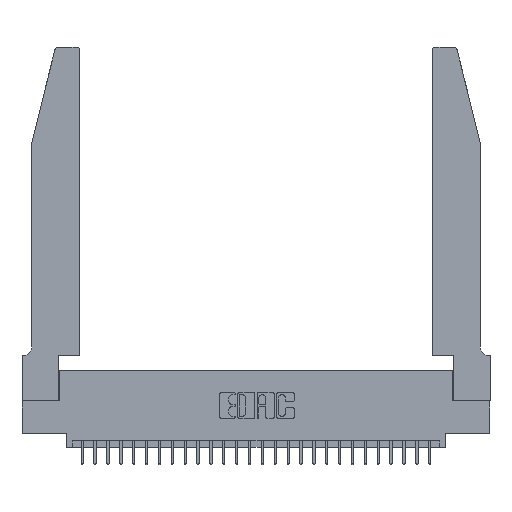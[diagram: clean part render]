
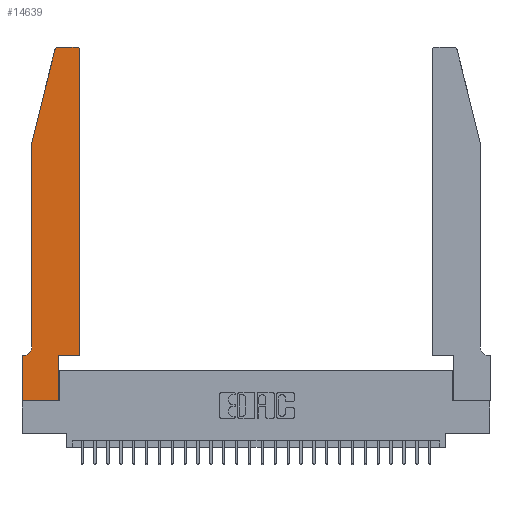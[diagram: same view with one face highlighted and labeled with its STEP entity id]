
A CAD part, top view. The second image highlights one B-rep face of the part: STEP entity #14639.
In plain terms, the highlighted planar face has unit normal (0, 0, 1).
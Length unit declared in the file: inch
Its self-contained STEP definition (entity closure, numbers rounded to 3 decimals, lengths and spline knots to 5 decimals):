
#9 = EDGE_CURVE ( 'NONE', #318, #7295, #23591, .T. ) ;
#57 = CARTESIAN_POINT ( 'NONE',  ( 0., 0.35, 0.37 ) ) ;
#318 = VERTEX_POINT ( 'NONE', #835 ) ;
#504 = DIRECTION ( 'NONE',  ( 1., 0., 0. ) ) ;
#835 = CARTESIAN_POINT ( 'NONE',  ( 0., 0.35, 0.37 ) ) ;
#884 = VERTEX_POINT ( 'NONE', #5884 ) ;
#1774 = LINE ( 'NONE', #19992, #11180 ) ;
#2488 = EDGE_CURVE ( 'NONE', #14502, #18545, #19866, .T. ) ;
#2671 = AXIS2_PLACEMENT_3D ( 'NONE', #21023, #7604, #20881 ) ;
#3238 = DIRECTION ( 'NONE',  ( 0., 1., 0. ) ) ;
#4235 = ORIENTED_EDGE ( 'NONE', *, *, #9, .T. ) ;
#4364 = DIRECTION ( 'NONE',  ( 1., 0., 0. ) ) ;
#4468 = ORIENTED_EDGE ( 'NONE', *, *, #12626, .T. ) ;
#4615 = EDGE_LOOP ( 'NONE', ( #11640, #15541, #27743, #25174, #7174, #15410, #4235, #6687, #4654, #4468, #18654, #24022 ) ) ;
#4654 = ORIENTED_EDGE ( 'NONE', *, *, #25054, .T. ) ;
#5324 = CARTESIAN_POINT ( 'NONE',  ( 0.4505, 0.35, 0.37 ) ) ;
#5884 = CARTESIAN_POINT ( 'NONE',  ( 0.0755, 2., 0.37 ) ) ;
#6075 = EDGE_CURVE ( 'NONE', #17084, #14502, #9820, .T. ) ;
#6185 = CARTESIAN_POINT ( 'NONE',  ( 0.4505, 2.72, 0.37 ) ) ;
#6214 = CARTESIAN_POINT ( 'NONE',  ( 0.0755, 2., 0.37 ) ) ;
#6383 = VERTEX_POINT ( 'NONE', #20259 ) ;
#6635 = CARTESIAN_POINT ( 'NONE',  ( 0.0055, 0.42, 0.37 ) ) ;
#6687 = ORIENTED_EDGE ( 'NONE', *, *, #10518, .T. ) ;
#6731 = VECTOR ( 'NONE', #17274, 39.37008 ) ;
#6787 = AXIS2_PLACEMENT_3D ( 'NONE', #57, #11114, #504 ) ;
#7174 = ORIENTED_EDGE ( 'NONE', *, *, #16550, .T. ) ;
#7295 = VERTEX_POINT ( 'NONE', #9009 ) ;
#7604 = DIRECTION ( 'NONE',  ( 0., 0., 1. ) ) ;
#8099 = CARTESIAN_POINT ( 'NONE',  ( 0.2865, 0.35, 0.37 ) ) ;
#8290 = LINE ( 'NONE', #14444, #14139 ) ;
#9009 = CARTESIAN_POINT ( 'NONE',  ( 0., 0., 0.37 ) ) ;
#9427 = VECTOR ( 'NONE', #4364, 39.37008 ) ;
#9759 = VERTEX_POINT ( 'NONE', #22353 ) ;
#9820 = LINE ( 'NONE', #20915, #17153 ) ;
#10478 = DIRECTION ( 'NONE',  ( -1., 0., 0. ) ) ;
#10518 = EDGE_CURVE ( 'NONE', #7295, #13391, #16001, .T. ) ;
#10576 = LINE ( 'NONE', #6214, #6731 ) ;
#10853 = DIRECTION ( 'NONE',  ( -1., 0., 0. ) ) ;
#11114 = DIRECTION ( 'NONE',  ( 0., 0., 1. ) ) ;
#11180 = VECTOR ( 'NONE', #22343, 39.37008 ) ;
#11543 = FACE_OUTER_BOUND ( 'NONE', #4615, .T. ) ;
#11640 = ORIENTED_EDGE ( 'NONE', *, *, #18376, .T. ) ;
#11825 = DIRECTION ( 'NONE',  ( 0., -1., 0. ) ) ;
#12626 = EDGE_CURVE ( 'NONE', #15548, #17084, #13453, .T. ) ;
#12737 = DIRECTION ( 'NONE',  ( 0., 0., -1. ) ) ;
#13391 = VERTEX_POINT ( 'NONE', #22506 ) ;
#13453 = LINE ( 'NONE', #26604, #26737 ) ;
#13742 = LINE ( 'NONE', #27337, #27738 ) ;
#13824 = CARTESIAN_POINT ( 'NONE',  ( 0., 0., 0.37 ) ) ;
#14139 = VECTOR ( 'NONE', #10478, 39.37008 ) ;
#14385 = DIRECTION ( 'NONE',  ( 1., 0., 0. ) ) ;
#14428 = CARTESIAN_POINT ( 'NONE',  ( 0.2865, 0.35, 0.37 ) ) ;
#14435 = CIRCLE ( 'NONE', #19531, 0.03 ) ;
#14444 = CARTESIAN_POINT ( 'NONE',  ( 0.0755, 0.35, 0.37 ) ) ;
#14502 = VERTEX_POINT ( 'NONE', #6185 ) ;
#14639 = ADVANCED_FACE ( 'NONE', ( #11543 ), #20466, .T. ) ;
#15410 = ORIENTED_EDGE ( 'NONE', *, *, #21966, .T. ) ;
#15460 = EDGE_CURVE ( 'NONE', #9759, #19875, #14435, .T. ) ;
#15541 = ORIENTED_EDGE ( 'NONE', *, *, #15460, .T. ) ;
#15548 = VERTEX_POINT ( 'NONE', #8099 ) ;
#16001 = LINE ( 'NONE', #13824, #9427 ) ;
#16056 = VECTOR ( 'NONE', #3238, 39.37008 ) ;
#16550 = EDGE_CURVE ( 'NONE', #20673, #6383, #27076, .T. ) ;
#16566 = DIRECTION ( 'NONE',  ( 0., 0., 1. ) ) ;
#17084 = VERTEX_POINT ( 'NONE', #5324 ) ;
#17153 = VECTOR ( 'NONE', #27508, 39.37008 ) ;
#17274 = DIRECTION ( 'NONE',  ( -0.239, -0.971, 0. ) ) ;
#18376 = EDGE_CURVE ( 'NONE', #18545, #9759, #1774, .T. ) ;
#18545 = VERTEX_POINT ( 'NONE', #20285 ) ;
#18654 = ORIENTED_EDGE ( 'NONE', *, *, #6075, .T. ) ;
#18769 = CARTESIAN_POINT ( 'NONE',  ( 0.284, 2.72, 0.37 ) ) ;
#19531 = AXIS2_PLACEMENT_3D ( 'NONE', #18769, #16566, #14385 ) ;
#19866 = CIRCLE ( 'NONE', #2671, 0.03 ) ;
#19875 = VERTEX_POINT ( 'NONE', #21846 ) ;
#19992 = CARTESIAN_POINT ( 'NONE',  ( 0.2605, 2.75, 0.37 ) ) ;
#20259 = CARTESIAN_POINT ( 'NONE',  ( 0.0055, 0.35, 0.37 ) ) ;
#20285 = CARTESIAN_POINT ( 'NONE',  ( 0.4205, 2.75, 0.37 ) ) ;
#20466 = PLANE ( 'NONE',  #6787 ) ;
#20673 = VERTEX_POINT ( 'NONE', #24156 ) ;
#20881 = DIRECTION ( 'NONE',  ( 1., 0., 0. ) ) ;
#20915 = CARTESIAN_POINT ( 'NONE',  ( 0.4505, 0.35, 0.37 ) ) ;
#20981 = CARTESIAN_POINT ( 'NONE',  ( 0., 0., 0.37 ) ) ;
#21023 = CARTESIAN_POINT ( 'NONE',  ( 0.4205, 2.72, 0.37 ) ) ;
#21846 = CARTESIAN_POINT ( 'NONE',  ( 0.25487, 2.72718, 0.37 ) ) ;
#21966 = EDGE_CURVE ( 'NONE', #6383, #318, #8290, .T. ) ;
#22343 = DIRECTION ( 'NONE',  ( -1., 0., 0. ) ) ;
#22353 = CARTESIAN_POINT ( 'NONE',  ( 0.284, 2.75, 0.37 ) ) ;
#22506 = CARTESIAN_POINT ( 'NONE',  ( 0.2865, 0., 0.37 ) ) ;
#23512 = VECTOR ( 'NONE', #27997, 39.37008 ) ;
#23591 = LINE ( 'NONE', #20981, #23512 ) ;
#24022 = ORIENTED_EDGE ( 'NONE', *, *, #2488, .T. ) ;
#24156 = CARTESIAN_POINT ( 'NONE',  ( 0.0755, 0.42, 0.37 ) ) ;
#24931 = EDGE_CURVE ( 'NONE', #884, #20673, #13742, .T. ) ;
#25054 = EDGE_CURVE ( 'NONE', #13391, #15548, #28548, .T. ) ;
#25104 = EDGE_CURVE ( 'NONE', #19875, #884, #10576, .T. ) ;
#25174 = ORIENTED_EDGE ( 'NONE', *, *, #24931, .T. ) ;
#26123 = AXIS2_PLACEMENT_3D ( 'NONE', #6635, #12737, #10853 ) ;
#26604 = CARTESIAN_POINT ( 'NONE',  ( 0.4505, 0.35, 0.37 ) ) ;
#26737 = VECTOR ( 'NONE', #27198, 39.37008 ) ;
#27076 = CIRCLE ( 'NONE', #26123, 0.07 ) ;
#27198 = DIRECTION ( 'NONE',  ( 1., 0., 0. ) ) ;
#27337 = CARTESIAN_POINT ( 'NONE',  ( 0.0755, 2., 0.37 ) ) ;
#27508 = DIRECTION ( 'NONE',  ( 0., 1., 0. ) ) ;
#27738 = VECTOR ( 'NONE', #11825, 39.37008 ) ;
#27743 = ORIENTED_EDGE ( 'NONE', *, *, #25104, .T. ) ;
#27997 = DIRECTION ( 'NONE',  ( 0., -1., 0. ) ) ;
#28548 = LINE ( 'NONE', #14428, #16056 ) ;
